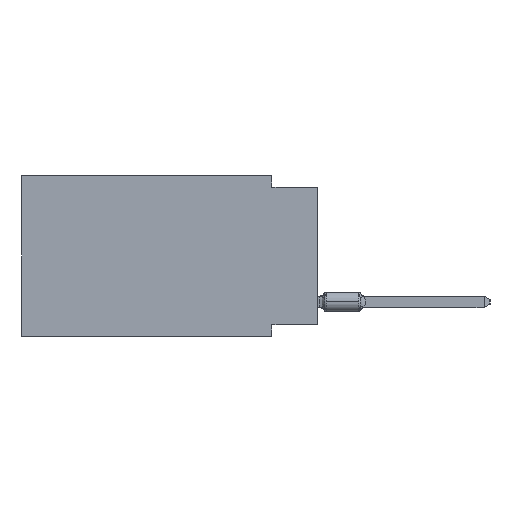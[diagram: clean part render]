
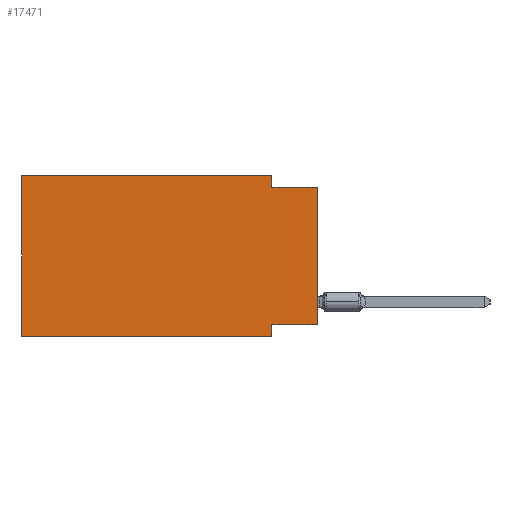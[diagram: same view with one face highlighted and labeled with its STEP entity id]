
A CAD part, left-side view. The second image highlights one B-rep face of the part: STEP entity #17471.
In plain terms, the highlighted planar face has unit normal (-1, 0, 0).
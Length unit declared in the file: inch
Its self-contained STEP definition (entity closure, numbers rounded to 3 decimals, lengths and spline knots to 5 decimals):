
#230 = LINE ( 'NONE', #17126, #19128 ) ;
#253 = AXIS2_PLACEMENT_3D ( 'NONE', #13858, #27022, #24811 ) ;
#1161 = VECTOR ( 'NONE', #14124, 39.37008 ) ;
#1232 = EDGE_CURVE ( 'NONE', #3902, #1285, #26864, .T. ) ;
#1285 = VERTEX_POINT ( 'NONE', #7730 ) ;
#3203 = VERTEX_POINT ( 'NONE', #24229 ) ;
#3247 = VERTEX_POINT ( 'NONE', #9668 ) ;
#3700 = LINE ( 'NONE', #12420, #17517 ) ;
#3849 = LINE ( 'NONE', #12293, #7793 ) ;
#3902 = VERTEX_POINT ( 'NONE', #17084 ) ;
#4255 = LINE ( 'NONE', #16714, #25549 ) ;
#4520 = VECTOR ( 'NONE', #16247, 39.37008 ) ;
#4654 = ORIENTED_EDGE ( 'NONE', *, *, #16260, .T. ) ;
#4815 = DIRECTION ( 'NONE',  ( 0., 0., 1. ) ) ;
#5277 = VERTEX_POINT ( 'NONE', #7137 ) ;
#5388 = ORIENTED_EDGE ( 'NONE', *, *, #14438, .F. ) ;
#5664 = DIRECTION ( 'NONE',  ( 0., -1., 0. ) ) ;
#5813 = EDGE_CURVE ( 'NONE', #3902, #20148, #7789, .T. ) ;
#7137 = CARTESIAN_POINT ( 'NONE',  ( 0., 0.1, 0. ) ) ;
#7497 = ORIENTED_EDGE ( 'NONE', *, *, #26429, .F. ) ;
#7730 = CARTESIAN_POINT ( 'NONE',  ( 0., 0., -0.025 ) ) ;
#7789 = LINE ( 'NONE', #22755, #4520 ) ;
#7793 = VECTOR ( 'NONE', #27240, 39.37008 ) ;
#7884 = LINE ( 'NONE', #18681, #1161 ) ;
#7899 = PLANE ( 'NONE',  #253 ) ;
#8485 = EDGE_CURVE ( 'NONE', #3247, #1285, #4255, .T. ) ;
#9668 = CARTESIAN_POINT ( 'NONE',  ( 0., 0.1, -0.025 ) ) ;
#11359 = DIRECTION ( 'NONE',  ( 0., 0., -1. ) ) ;
#11608 = ORIENTED_EDGE ( 'NONE', *, *, #8485, .F. ) ;
#11725 = EDGE_LOOP ( 'NONE', ( #11848, #11608, #23088, #21809, #7497, #4654, #5388, #19741 ) ) ;
#11848 = ORIENTED_EDGE ( 'NONE', *, *, #1232, .T. ) ;
#11921 = FACE_OUTER_BOUND ( 'NONE', #11725, .T. ) ;
#12022 = DIRECTION ( 'NONE',  ( 0., 0., 1. ) ) ;
#12293 = CARTESIAN_POINT ( 'NONE',  ( 0., 0.1, -0.35 ) ) ;
#12420 = CARTESIAN_POINT ( 'NONE',  ( 0., 0.645, -0.35 ) ) ;
#13012 = VERTEX_POINT ( 'NONE', #27232 ) ;
#13858 = CARTESIAN_POINT ( 'NONE',  ( 0., 0.645, 0. ) ) ;
#14124 = DIRECTION ( 'NONE',  ( 0., -1., 0. ) ) ;
#14438 = EDGE_CURVE ( 'NONE', #20148, #17849, #3849, .T. ) ;
#15055 = DIRECTION ( 'NONE',  ( 0., -1., 0. ) ) ;
#16247 = DIRECTION ( 'NONE',  ( 0., 1., 0. ) ) ;
#16260 = EDGE_CURVE ( 'NONE', #3203, #17849, #3700, .T. ) ;
#16714 = CARTESIAN_POINT ( 'NONE',  ( 0., 0., -0.025 ) ) ;
#17084 = CARTESIAN_POINT ( 'NONE',  ( 0., 0., -0.325 ) ) ;
#17126 = CARTESIAN_POINT ( 'NONE',  ( 0., 0.645, 0. ) ) ;
#17180 = CARTESIAN_POINT ( 'NONE',  ( 0., 0.1, -0.325 ) ) ;
#17471 = ADVANCED_FACE ( 'NONE', ( #11921 ), #7899, .F. ) ;
#17517 = VECTOR ( 'NONE', #5664, 39.37008 ) ;
#17849 = VERTEX_POINT ( 'NONE', #19044 ) ;
#18681 = CARTESIAN_POINT ( 'NONE',  ( 0., 0.645, 0. ) ) ;
#19044 = CARTESIAN_POINT ( 'NONE',  ( 0., 0.1, -0.35 ) ) ;
#19128 = VECTOR ( 'NONE', #4815, 39.37008 ) ;
#19741 = ORIENTED_EDGE ( 'NONE', *, *, #5813, .F. ) ;
#20148 = VERTEX_POINT ( 'NONE', #17180 ) ;
#20207 = EDGE_CURVE ( 'NONE', #5277, #3247, #26185, .T. ) ;
#21493 = VECTOR ( 'NONE', #12022, 39.37008 ) ;
#21571 = EDGE_CURVE ( 'NONE', #13012, #5277, #7884, .T. ) ;
#21809 = ORIENTED_EDGE ( 'NONE', *, *, #21571, .F. ) ;
#22407 = VECTOR ( 'NONE', #11359, 39.37008 ) ;
#22755 = CARTESIAN_POINT ( 'NONE',  ( 0., 0., -0.325 ) ) ;
#23088 = ORIENTED_EDGE ( 'NONE', *, *, #20207, .F. ) ;
#24102 = CARTESIAN_POINT ( 'NONE',  ( 0., 0.1, 0. ) ) ;
#24229 = CARTESIAN_POINT ( 'NONE',  ( 0., 0.645, -0.35 ) ) ;
#24374 = CARTESIAN_POINT ( 'NONE',  ( 0., 0., 0. ) ) ;
#24811 = DIRECTION ( 'NONE',  ( 0., 0., -1. ) ) ;
#25549 = VECTOR ( 'NONE', #15055, 39.37008 ) ;
#26185 = LINE ( 'NONE', #24102, #22407 ) ;
#26429 = EDGE_CURVE ( 'NONE', #3203, #13012, #230, .T. ) ;
#26864 = LINE ( 'NONE', #24374, #21493 ) ;
#27022 = DIRECTION ( 'NONE',  ( 1., 0., 0. ) ) ;
#27232 = CARTESIAN_POINT ( 'NONE',  ( 0., 0.645, 0. ) ) ;
#27240 = DIRECTION ( 'NONE',  ( 0., 0., -1. ) ) ;
